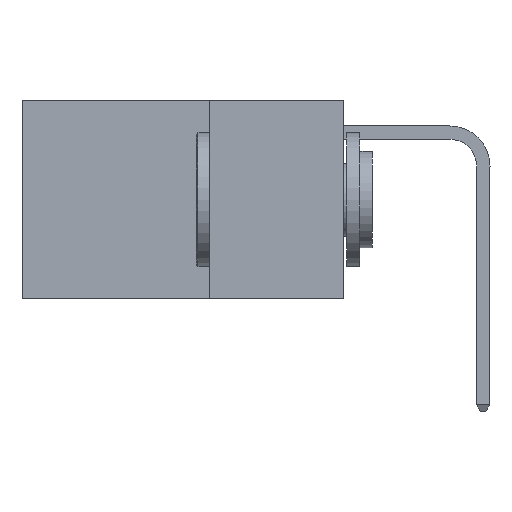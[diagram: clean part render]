
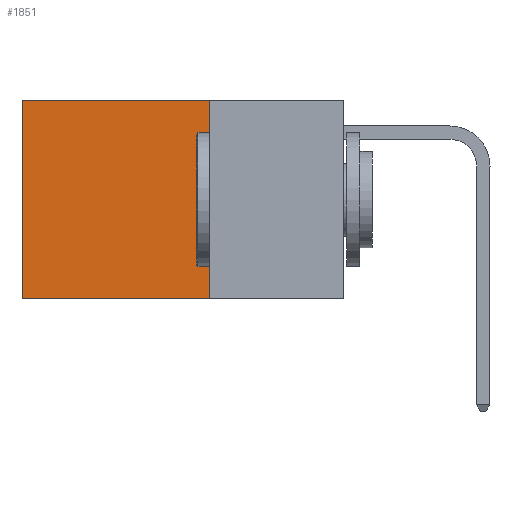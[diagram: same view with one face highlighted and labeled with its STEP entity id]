
A CAD part, left-side view. The second image highlights one B-rep face of the part: STEP entity #1851.
In plain terms, the highlighted planar face has unit normal (-1, 0, 0).
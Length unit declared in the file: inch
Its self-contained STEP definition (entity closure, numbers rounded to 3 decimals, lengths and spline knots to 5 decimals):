
#843 = ORIENTED_EDGE ( 'NONE', *, *, #1476, .T. ) ;
#878 = ORIENTED_EDGE ( 'NONE', *, *, #1334, .F. ) ;
#887 = ORIENTED_EDGE ( 'NONE', *, *, #5044, .F. ) ;
#990 = ORIENTED_EDGE ( 'NONE', *, *, #9271, .T. ) ;
#1061 = LINE ( 'NONE', #4318, #7299 ) ;
#1329 = EDGE_LOOP ( 'NONE', ( #843, #878, #887, #990 ) ) ;
#1334 = EDGE_CURVE ( 'NONE', #4242, #3555, #10520, .T. ) ;
#1476 = EDGE_CURVE ( 'NONE', #4744, #3555, #4989, .T. ) ;
#1851 = ADVANCED_FACE ( 'NONE', ( #9567 ), #6467, .F. ) ;
#2540 = CARTESIAN_POINT ( 'NONE',  ( 0.2625, 0.25, 0. ) ) ;
#2657 = DIRECTION ( 'NONE',  ( 0., 0., -1. ) ) ;
#3555 = VERTEX_POINT ( 'NONE', #7845 ) ;
#4242 = VERTEX_POINT ( 'NONE', #10024 ) ;
#4318 = CARTESIAN_POINT ( 'NONE',  ( 0.2625, 0.25, 0. ) ) ;
#4354 = VECTOR ( 'NONE', #9048, 39.37008 ) ;
#4438 = CARTESIAN_POINT ( 'NONE',  ( 0.2625, 0.25, 0. ) ) ;
#4744 = VERTEX_POINT ( 'NONE', #5963 ) ;
#4989 = LINE ( 'NONE', #8484, #7230 ) ;
#5044 = EDGE_CURVE ( 'NONE', #9339, #4242, #7787, .T. ) ;
#5137 = AXIS2_PLACEMENT_3D ( 'NONE', #6438, #6409, #6395 ) ;
#5596 = VECTOR ( 'NONE', #2657, 39.37008 ) ;
#5963 = CARTESIAN_POINT ( 'NONE',  ( 0.2625, 0.6, 0. ) ) ;
#5994 = DIRECTION ( 'NONE',  ( 0., 1., 0. ) ) ;
#6395 = DIRECTION ( 'NONE',  ( 0., 0., -1. ) ) ;
#6409 = DIRECTION ( 'NONE',  ( 1., 0., 0. ) ) ;
#6438 = CARTESIAN_POINT ( 'NONE',  ( 0.2625, 0.25, 0. ) ) ;
#6467 = PLANE ( 'NONE',  #5137 ) ;
#7230 = VECTOR ( 'NONE', #8446, 39.37008 ) ;
#7299 = VECTOR ( 'NONE', #5994, 39.37008 ) ;
#7787 = LINE ( 'NONE', #2540, #5596 ) ;
#7845 = CARTESIAN_POINT ( 'NONE',  ( 0.2625, 0.6, -0.37 ) ) ;
#8446 = DIRECTION ( 'NONE',  ( 0., 0., -1. ) ) ;
#8484 = CARTESIAN_POINT ( 'NONE',  ( 0.2625, 0.6, 0. ) ) ;
#9048 = DIRECTION ( 'NONE',  ( 0., 1., 0. ) ) ;
#9085 = CARTESIAN_POINT ( 'NONE',  ( 0.2625, 0.25, -0.37 ) ) ;
#9271 = EDGE_CURVE ( 'NONE', #9339, #4744, #1061, .T. ) ;
#9339 = VERTEX_POINT ( 'NONE', #4438 ) ;
#9567 = FACE_OUTER_BOUND ( 'NONE', #1329, .T. ) ;
#10024 = CARTESIAN_POINT ( 'NONE',  ( 0.2625, 0.25, -0.37 ) ) ;
#10520 = LINE ( 'NONE', #9085, #4354 ) ;
